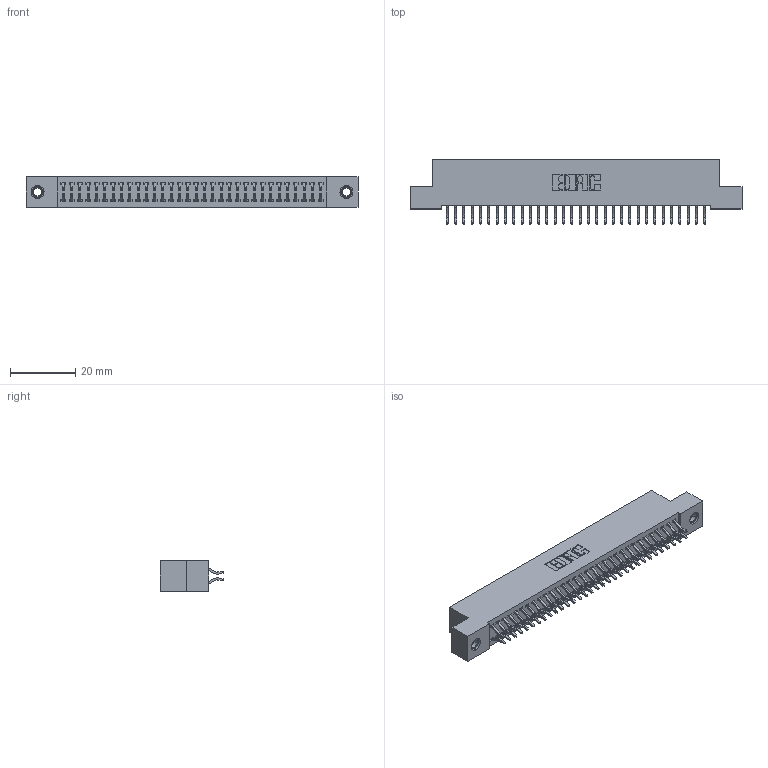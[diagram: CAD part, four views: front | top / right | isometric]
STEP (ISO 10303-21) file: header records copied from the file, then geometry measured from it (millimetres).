
FILE_DESCRIPTION (( 'STEP AP203' ), '1' );
FILE_NAME ('392-064-556-207.STEP', '2018-08-17T21:51:46', ( '' ), ( '' ), 'SwSTEP 2.0', 'SolidWorks 2016', '' );
FILE_SCHEMA (( 'CONFIG_CONTROL_DESIGN' ));
Length unit declared in the file: inch
Products named in the file (4): 342 Part_TI; 345-292-001_556 Tail; 345-250-001_345-250-005-103; 392-064-556-207
Assembly tree (67 placements, depth 2):
  392-064-556-207
    342 Part_TI
    345-292-001_556 Tail  x64
    345-250-001_345-250-005-103  x2
Bounding box: 101.6 x 19.58 x 9.4 mm (x, y, z)
Volume: 9067.1 mm3; surface area: 14476.3 mm2
Topology: 67 solids, 67 shells, 3882 faces, 11507 edges, 7578 vertices
Faces by surface type: plane 2658, cylinder 1208, cone 12, torus 4
Entity records: 23154 total; most frequent: CARTESIAN_POINT 3845, ORIENTED_EDGE 3762, DIRECTION 3323, EDGE_CURVE 1881, LINE 1725, VECTOR 1725, VERTEX_POINT 1248, AXIS2_PLACEMENT_3D 799
